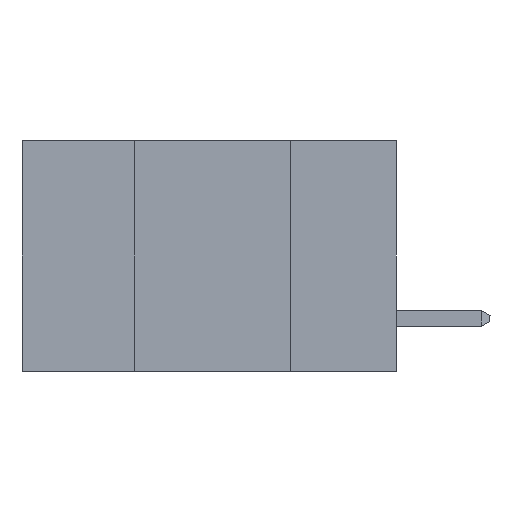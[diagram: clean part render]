
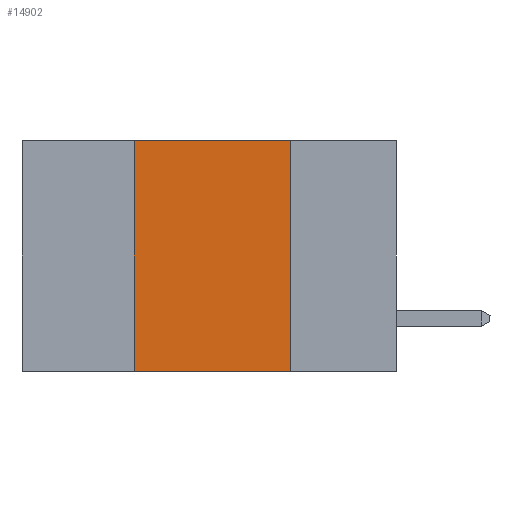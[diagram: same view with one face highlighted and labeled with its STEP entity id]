
A CAD part, left-side view. The second image highlights one B-rep face of the part: STEP entity #14902.
In plain terms, the highlighted planar face has unit normal (-1, 0, 0).
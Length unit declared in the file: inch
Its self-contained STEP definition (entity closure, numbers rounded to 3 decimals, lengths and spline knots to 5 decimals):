
#339 = ORIENTED_EDGE ( 'NONE', *, *, #5614, .T. ) ;
#1514 = ORIENTED_EDGE ( 'NONE', *, *, #2216, .F. ) ;
#2100 = DIRECTION ( 'NONE',  ( 0., -1., 0. ) ) ;
#2216 = EDGE_CURVE ( 'NONE', #15349, #3928, #12016, .T. ) ;
#3073 = CARTESIAN_POINT ( 'NONE',  ( 0., 0.42, -0.37 ) ) ;
#3671 = AXIS2_PLACEMENT_3D ( 'NONE', #7822, #15337, #4126 ) ;
#3697 = VECTOR ( 'NONE', #8946, 39.37008 ) ;
#3928 = VERTEX_POINT ( 'NONE', #14985 ) ;
#4044 = VERTEX_POINT ( 'NONE', #15468 ) ;
#4126 = DIRECTION ( 'NONE',  ( 0., 0., -1. ) ) ;
#5296 = CARTESIAN_POINT ( 'NONE',  ( 0., 0.6, 0. ) ) ;
#5323 = CARTESIAN_POINT ( 'NONE',  ( 0., 0.17, -0.37 ) ) ;
#5614 = EDGE_CURVE ( 'NONE', #15349, #10556, #5892, .T. ) ;
#5883 = EDGE_CURVE ( 'NONE', #3928, #4044, #10407, .T. ) ;
#5892 = LINE ( 'NONE', #15971, #12342 ) ;
#6630 = DIRECTION ( 'NONE',  ( 0., -1., 0. ) ) ;
#7441 = ORIENTED_EDGE ( 'NONE', *, *, #5883, .F. ) ;
#7448 = LINE ( 'NONE', #15132, #3697 ) ;
#7822 = CARTESIAN_POINT ( 'NONE',  ( 0., 0.6, 0. ) ) ;
#8113 = EDGE_LOOP ( 'NONE', ( #12426, #7441, #1514, #339 ) ) ;
#8173 = DIRECTION ( 'NONE',  ( 0., 0., 1. ) ) ;
#8946 = DIRECTION ( 'NONE',  ( 0., 0., -1. ) ) ;
#9310 = PLANE ( 'NONE',  #3671 ) ;
#9874 = CARTESIAN_POINT ( 'NONE',  ( 0., 0.42, -0.37 ) ) ;
#10407 = LINE ( 'NONE', #5296, #13072 ) ;
#10556 = VERTEX_POINT ( 'NONE', #5323 ) ;
#11672 = FACE_OUTER_BOUND ( 'NONE', #8113, .T. ) ;
#12016 = LINE ( 'NONE', #3073, #14974 ) ;
#12342 = VECTOR ( 'NONE', #2100, 39.37008 ) ;
#12426 = ORIENTED_EDGE ( 'NONE', *, *, #15977, .F. ) ;
#13072 = VECTOR ( 'NONE', #6630, 39.37008 ) ;
#14902 = ADVANCED_FACE ( 'NONE', ( #11672 ), #9310, .F. ) ;
#14974 = VECTOR ( 'NONE', #8173, 39.37008 ) ;
#14985 = CARTESIAN_POINT ( 'NONE',  ( 0., 0.42, 0. ) ) ;
#15132 = CARTESIAN_POINT ( 'NONE',  ( 0., 0.17, -0.37 ) ) ;
#15337 = DIRECTION ( 'NONE',  ( 1., 0., 0. ) ) ;
#15349 = VERTEX_POINT ( 'NONE', #9874 ) ;
#15468 = CARTESIAN_POINT ( 'NONE',  ( 0., 0.17, 0. ) ) ;
#15971 = CARTESIAN_POINT ( 'NONE',  ( 0., 0.6, -0.37 ) ) ;
#15977 = EDGE_CURVE ( 'NONE', #4044, #10556, #7448, .T. ) ;
